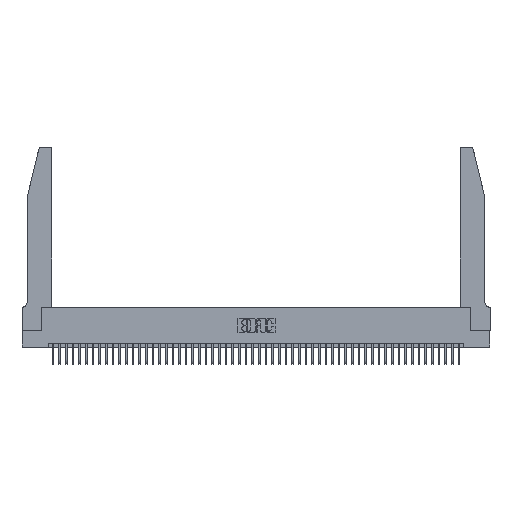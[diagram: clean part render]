
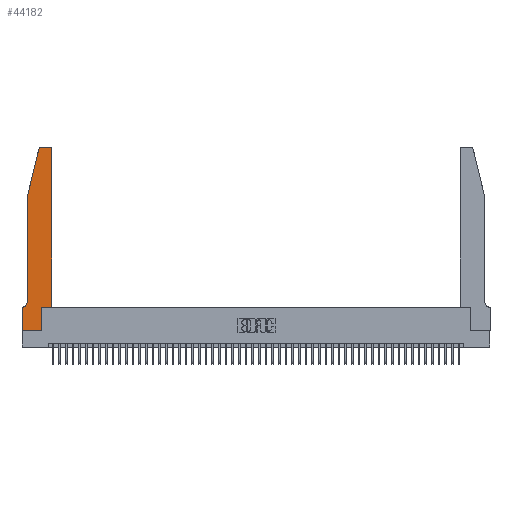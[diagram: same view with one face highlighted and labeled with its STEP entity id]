
A CAD part, top view. The second image highlights one B-rep face of the part: STEP entity #44182.
In plain terms, the highlighted planar face has unit normal (0, 0, 1).
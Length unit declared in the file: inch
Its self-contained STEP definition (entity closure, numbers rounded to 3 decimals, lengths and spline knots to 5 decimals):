
#1547 = PLANE ( 'NONE',  #17777 ) ;
#3043 = LINE ( 'NONE', #42244, #23439 ) ;
#3116 = CIRCLE ( 'NONE', #3607, 0.03 ) ;
#3160 = EDGE_CURVE ( 'NONE', #4740, #21057, #6899, .T. ) ;
#3607 = AXIS2_PLACEMENT_3D ( 'NONE', #41713, #17576, #45736 ) ;
#3882 = CARTESIAN_POINT ( 'NONE',  ( 0.0055, 0.42, 0.37 ) ) ;
#4214 = ORIENTED_EDGE ( 'NONE', *, *, #43489, .T. ) ;
#4740 = VERTEX_POINT ( 'NONE', #51470 ) ;
#4988 = CARTESIAN_POINT ( 'NONE',  ( 0.0755, 2., 0.37 ) ) ;
#5063 = CARTESIAN_POINT ( 'NONE',  ( 0.4205, 2.72, 0.37 ) ) ;
#5588 = EDGE_CURVE ( 'NONE', #50053, #13851, #9840, .T. ) ;
#5922 = CARTESIAN_POINT ( 'NONE',  ( 0., 0., 0.37 ) ) ;
#6563 = ORIENTED_EDGE ( 'NONE', *, *, #19056, .T. ) ;
#6899 = LINE ( 'NONE', #4988, #48584 ) ;
#7964 = EDGE_CURVE ( 'NONE', #21057, #50053, #21039, .T. ) ;
#8021 = DIRECTION ( 'NONE',  ( -1., 0., 0. ) ) ;
#8518 = CARTESIAN_POINT ( 'NONE',  ( 0.4205, 2.75, 0.37 ) ) ;
#9019 = CARTESIAN_POINT ( 'NONE',  ( 0.0755, 2., 0.37 ) ) ;
#9207 = DIRECTION ( 'NONE',  ( 1., 0., 0. ) ) ;
#9606 = VERTEX_POINT ( 'NONE', #27539 ) ;
#9746 = ORIENTED_EDGE ( 'NONE', *, *, #13148, .T. ) ;
#9840 = CIRCLE ( 'NONE', #47736, 0.07 ) ;
#10083 = DIRECTION ( 'NONE',  ( 0., -1., 0. ) ) ;
#10372 = CARTESIAN_POINT ( 'NONE',  ( 0.0755, 2., 0.37 ) ) ;
#10730 = EDGE_CURVE ( 'NONE', #9606, #41748, #44127, .T. ) ;
#13148 = EDGE_CURVE ( 'NONE', #31401, #34079, #38856, .T. ) ;
#13309 = AXIS2_PLACEMENT_3D ( 'NONE', #5063, #33468, #9207 ) ;
#13851 = VERTEX_POINT ( 'NONE', #15670 ) ;
#15087 = EDGE_CURVE ( 'NONE', #23137, #17509, #3043, .T. ) ;
#15670 = CARTESIAN_POINT ( 'NONE',  ( 0.0055, 0.35, 0.37 ) ) ;
#15936 = ORIENTED_EDGE ( 'NONE', *, *, #26399, .T. ) ;
#16073 = FACE_OUTER_BOUND ( 'NONE', #45132, .T. ) ;
#16748 = DIRECTION ( 'NONE',  ( 1., 0., 0. ) ) ;
#16780 = VECTOR ( 'NONE', #50066, 39.37008 ) ;
#17509 = VERTEX_POINT ( 'NONE', #17537 ) ;
#17537 = CARTESIAN_POINT ( 'NONE',  ( 0.284, 2.75, 0.37 ) ) ;
#17576 = DIRECTION ( 'NONE',  ( 0., 0., 1. ) ) ;
#17777 = AXIS2_PLACEMENT_3D ( 'NONE', #18006, #46173, #22098 ) ;
#18006 = CARTESIAN_POINT ( 'NONE',  ( 0., 0.35, 0.37 ) ) ;
#18130 = DIRECTION ( 'NONE',  ( -1., 0., 0. ) ) ;
#18529 = VECTOR ( 'NONE', #33103, 39.37008 ) ;
#18782 = VECTOR ( 'NONE', #22914, 39.37008 ) ;
#18865 = CARTESIAN_POINT ( 'NONE',  ( 0.0755, 0.35, 0.37 ) ) ;
#19056 = EDGE_CURVE ( 'NONE', #34079, #23137, #40733, .T. ) ;
#19069 = CARTESIAN_POINT ( 'NONE',  ( 0.2865, 0.35, 0.37 ) ) ;
#19283 = CARTESIAN_POINT ( 'NONE',  ( 0.4505, 0.35, 0.37 ) ) ;
#19963 = VECTOR ( 'NONE', #31456, 39.37008 ) ;
#20686 = DIRECTION ( 'NONE',  ( 1., 0., 0. ) ) ;
#20693 = LINE ( 'NONE', #24691, #51482 ) ;
#21039 = LINE ( 'NONE', #9019, #18529 ) ;
#21057 = VERTEX_POINT ( 'NONE', #10372 ) ;
#21203 = ORIENTED_EDGE ( 'NONE', *, *, #15087, .T. ) ;
#22098 = DIRECTION ( 'NONE',  ( 1., 0., 0. ) ) ;
#22103 = CARTESIAN_POINT ( 'NONE',  ( 0.4505, 0.35, 0.37 ) ) ;
#22914 = DIRECTION ( 'NONE',  ( -1., 0., 0. ) ) ;
#23137 = VERTEX_POINT ( 'NONE', #8518 ) ;
#23439 = VECTOR ( 'NONE', #18130, 39.37008 ) ;
#23667 = ORIENTED_EDGE ( 'NONE', *, *, #5588, .T. ) ;
#23991 = VECTOR ( 'NONE', #10083, 39.37008 ) ;
#24427 = LINE ( 'NONE', #18865, #18782 ) ;
#24691 = CARTESIAN_POINT ( 'NONE',  ( 0.4505, 0.35, 0.37 ) ) ;
#26399 = EDGE_CURVE ( 'NONE', #41748, #27759, #47311, .T. ) ;
#26952 = ORIENTED_EDGE ( 'NONE', *, *, #42515, .T. ) ;
#27539 = CARTESIAN_POINT ( 'NONE',  ( 0., 0.35, 0.37 ) ) ;
#27562 = ORIENTED_EDGE ( 'NONE', *, *, #7964, .T. ) ;
#27759 = VERTEX_POINT ( 'NONE', #38398 ) ;
#31401 = VERTEX_POINT ( 'NONE', #22103 ) ;
#31456 = DIRECTION ( 'NONE',  ( 0., 1., 0. ) ) ;
#32311 = DIRECTION ( 'NONE',  ( 0., 0., -1. ) ) ;
#32688 = CARTESIAN_POINT ( 'NONE',  ( 0., 0., 0.37 ) ) ;
#33103 = DIRECTION ( 'NONE',  ( 0., -1., 0. ) ) ;
#33468 = DIRECTION ( 'NONE',  ( 0., 0., 1. ) ) ;
#34079 = VERTEX_POINT ( 'NONE', #43586 ) ;
#35874 = ORIENTED_EDGE ( 'NONE', *, *, #3160, .T. ) ;
#36239 = CARTESIAN_POINT ( 'NONE',  ( 0., 0., 0.37 ) ) ;
#37450 = DIRECTION ( 'NONE',  ( -0.239, -0.971, 0. ) ) ;
#38398 = CARTESIAN_POINT ( 'NONE',  ( 0.2865, 0., 0.37 ) ) ;
#38856 = LINE ( 'NONE', #19283, #19963 ) ;
#39426 = EDGE_CURVE ( 'NONE', #17509, #4740, #3116, .T. ) ;
#40733 = CIRCLE ( 'NONE', #13309, 0.03 ) ;
#41713 = CARTESIAN_POINT ( 'NONE',  ( 0.284, 2.72, 0.37 ) ) ;
#41748 = VERTEX_POINT ( 'NONE', #36239 ) ;
#41774 = ORIENTED_EDGE ( 'NONE', *, *, #39426, .T. ) ;
#41908 = ORIENTED_EDGE ( 'NONE', *, *, #10730, .T. ) ;
#42013 = CARTESIAN_POINT ( 'NONE',  ( 0.2865, 0.35, 0.37 ) ) ;
#42244 = CARTESIAN_POINT ( 'NONE',  ( 0.2605, 2.75, 0.37 ) ) ;
#42515 = EDGE_CURVE ( 'NONE', #49338, #31401, #20693, .T. ) ;
#42890 = EDGE_CURVE ( 'NONE', #13851, #9606, #24427, .T. ) ;
#43489 = EDGE_CURVE ( 'NONE', #27759, #49338, #50129, .T. ) ;
#43586 = CARTESIAN_POINT ( 'NONE',  ( 0.4505, 2.72, 0.37 ) ) ;
#44127 = LINE ( 'NONE', #5922, #23991 ) ;
#44182 = ADVANCED_FACE ( 'NONE', ( #16073 ), #1547, .T. ) ;
#45132 = EDGE_LOOP ( 'NONE', ( #21203, #41774, #35874, #27562, #23667, #50192, #41908, #15936, #4214, #26952, #9746, #6563 ) ) ;
#45736 = DIRECTION ( 'NONE',  ( 1., 0., 0. ) ) ;
#46043 = VECTOR ( 'NONE', #20686, 39.37008 ) ;
#46173 = DIRECTION ( 'NONE',  ( 0., 0., 1. ) ) ;
#47311 = LINE ( 'NONE', #32688, #46043 ) ;
#47736 = AXIS2_PLACEMENT_3D ( 'NONE', #3882, #32311, #8021 ) ;
#48584 = VECTOR ( 'NONE', #37450, 39.37008 ) ;
#49338 = VERTEX_POINT ( 'NONE', #19069 ) ;
#50053 = VERTEX_POINT ( 'NONE', #52018 ) ;
#50066 = DIRECTION ( 'NONE',  ( 0., 1., 0. ) ) ;
#50129 = LINE ( 'NONE', #42013, #16780 ) ;
#50192 = ORIENTED_EDGE ( 'NONE', *, *, #42890, .T. ) ;
#51470 = CARTESIAN_POINT ( 'NONE',  ( 0.25487, 2.72718, 0.37 ) ) ;
#51482 = VECTOR ( 'NONE', #16748, 39.37008 ) ;
#52018 = CARTESIAN_POINT ( 'NONE',  ( 0.0755, 0.42, 0.37 ) ) ;
